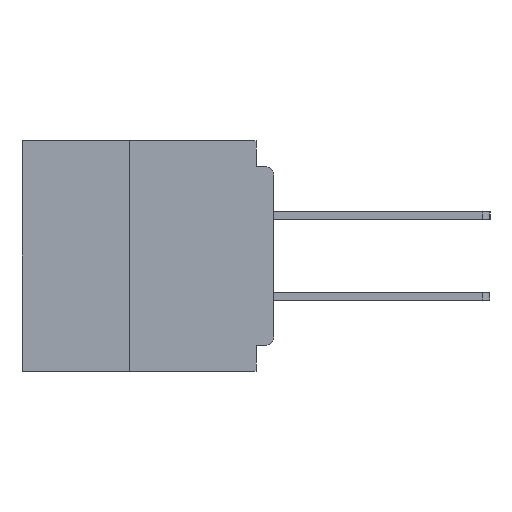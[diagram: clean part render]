
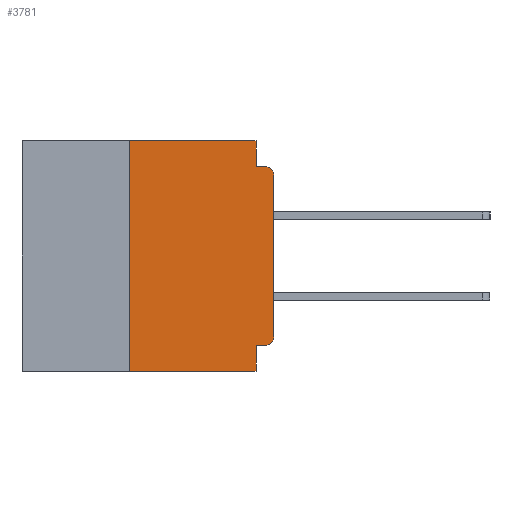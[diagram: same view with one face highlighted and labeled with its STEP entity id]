
A CAD part, left-side view. The second image highlights one B-rep face of the part: STEP entity #3781.
In plain terms, the highlighted planar face has unit normal (-1, 0, 0).
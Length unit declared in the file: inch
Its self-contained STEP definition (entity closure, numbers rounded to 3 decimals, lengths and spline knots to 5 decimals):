
#475 = LINE ( 'NONE', #21800, #40714 ) ;
#983 = DIRECTION ( 'NONE',  ( 0., -1., 0. ) ) ;
#988 = ORIENTED_EDGE ( 'NONE', *, *, #8666, .T. ) ;
#1054 = ORIENTED_EDGE ( 'NONE', *, *, #17307, .T. ) ;
#1255 = DIRECTION ( 'NONE',  ( 0., 0., -1. ) ) ;
#1446 = CARTESIAN_POINT ( 'NONE',  ( 0., 0.015, -0.34 ) ) ;
#1622 = LINE ( 'NONE', #14674, #27737 ) ;
#2168 = VERTEX_POINT ( 'NONE', #23121 ) ;
#2223 = EDGE_CURVE ( 'NONE', #4443, #34840, #23744, .T. ) ;
#2476 = ORIENTED_EDGE ( 'NONE', *, *, #20260, .F. ) ;
#3749 = CARTESIAN_POINT ( 'NONE',  ( 0., 0.031, -0.4 ) ) ;
#3781 = ADVANCED_FACE ( 'NONE', ( #30704 ), #23055, .F. ) ;
#4443 = VERTEX_POINT ( 'NONE', #14355 ) ;
#4814 = DIRECTION ( 'NONE',  ( 0., 0., -1. ) ) ;
#6836 = EDGE_CURVE ( 'NONE', #39723, #20368, #28505, .T. ) ;
#7075 = VERTEX_POINT ( 'NONE', #12648 ) ;
#7151 = AXIS2_PLACEMENT_3D ( 'NONE', #22767, #22483, #21456 ) ;
#8666 = EDGE_CURVE ( 'NONE', #13866, #19477, #31047, .T. ) ;
#10092 = VECTOR ( 'NONE', #23345, 39.37008 ) ;
#10559 = CIRCLE ( 'NONE', #15120, 0.015 ) ;
#12331 = VECTOR ( 'NONE', #38839, 39.37008 ) ;
#12599 = CARTESIAN_POINT ( 'NONE',  ( 0., 0.031, -0.045 ) ) ;
#12648 = CARTESIAN_POINT ( 'NONE',  ( 0., 0.015, -0.045 ) ) ;
#12701 = VERTEX_POINT ( 'NONE', #32894 ) ;
#13866 = VERTEX_POINT ( 'NONE', #36675 ) ;
#14355 = CARTESIAN_POINT ( 'NONE',  ( 0., 0., -0.34 ) ) ;
#14674 = CARTESIAN_POINT ( 'NONE',  ( 0., 0.25, -0.4 ) ) ;
#15120 = AXIS2_PLACEMENT_3D ( 'NONE', #1446, #24380, #4814 ) ;
#16251 = CARTESIAN_POINT ( 'NONE',  ( 0., 0.437, 0. ) ) ;
#17265 = EDGE_LOOP ( 'NONE', ( #40569, #27535, #2476, #29593, #20428, #24034, #988, #24592, #29224, #1054 ) ) ;
#17307 = EDGE_CURVE ( 'NONE', #2168, #4443, #10559, .T. ) ;
#17409 = CARTESIAN_POINT ( 'NONE',  ( 0., 0.437, -0.4 ) ) ;
#17545 = EDGE_CURVE ( 'NONE', #2168, #30224, #33842, .T. ) ;
#17609 = DIRECTION ( 'NONE',  ( 0., 0., 1. ) ) ;
#17804 = CARTESIAN_POINT ( 'NONE',  ( 0., 0., 0. ) ) ;
#18742 = LINE ( 'NONE', #3749, #10092 ) ;
#19477 = VERTEX_POINT ( 'NONE', #32264 ) ;
#20260 = EDGE_CURVE ( 'NONE', #20368, #7075, #475, .T. ) ;
#20368 = VERTEX_POINT ( 'NONE', #12599 ) ;
#20428 = ORIENTED_EDGE ( 'NONE', *, *, #30050, .F. ) ;
#20446 = CARTESIAN_POINT ( 'NONE',  ( 0., 0.031, -0.355 ) ) ;
#20901 = DIRECTION ( 'NONE',  ( -1., 0., 0. ) ) ;
#21456 = DIRECTION ( 'NONE',  ( 0., 0., -1. ) ) ;
#21800 = CARTESIAN_POINT ( 'NONE',  ( 0., 0., -0.045 ) ) ;
#21947 = LINE ( 'NONE', #16251, #12331 ) ;
#22402 = VECTOR ( 'NONE', #983, 39.37008 ) ;
#22483 = DIRECTION ( 'NONE',  ( 1., 0., 0. ) ) ;
#22767 = CARTESIAN_POINT ( 'NONE',  ( 0., 0.437, 0. ) ) ;
#23055 = PLANE ( 'NONE',  #7151 ) ;
#23121 = CARTESIAN_POINT ( 'NONE',  ( 0., 0.015, -0.355 ) ) ;
#23345 = DIRECTION ( 'NONE',  ( 0., 0., -1. ) ) ;
#23744 = LINE ( 'NONE', #17804, #33331 ) ;
#24034 = ORIENTED_EDGE ( 'NONE', *, *, #26545, .F. ) ;
#24218 = AXIS2_PLACEMENT_3D ( 'NONE', #40230, #20901, #1255 ) ;
#24380 = DIRECTION ( 'NONE',  ( -1., 0., 0. ) ) ;
#24592 = ORIENTED_EDGE ( 'NONE', *, *, #31867, .F. ) ;
#25498 = CARTESIAN_POINT ( 'NONE',  ( 0., 0., -0.355 ) ) ;
#26545 = EDGE_CURVE ( 'NONE', #13866, #12701, #1622, .T. ) ;
#27535 = ORIENTED_EDGE ( 'NONE', *, *, #40414, .T. ) ;
#27684 = CARTESIAN_POINT ( 'NONE',  ( 0., 0.031, 0. ) ) ;
#27737 = VECTOR ( 'NONE', #37281, 39.37008 ) ;
#28505 = LINE ( 'NONE', #27684, #36041 ) ;
#29224 = ORIENTED_EDGE ( 'NONE', *, *, #17545, .F. ) ;
#29593 = ORIENTED_EDGE ( 'NONE', *, *, #6836, .F. ) ;
#29956 = CARTESIAN_POINT ( 'NONE',  ( 0., 0., -0.06 ) ) ;
#30050 = EDGE_CURVE ( 'NONE', #12701, #39723, #21947, .T. ) ;
#30224 = VERTEX_POINT ( 'NONE', #20446 ) ;
#30322 = CIRCLE ( 'NONE', #24218, 0.015 ) ;
#30704 = FACE_OUTER_BOUND ( 'NONE', #17265, .T. ) ;
#31047 = LINE ( 'NONE', #17409, #22402 ) ;
#31867 = EDGE_CURVE ( 'NONE', #30224, #19477, #18742, .T. ) ;
#32004 = DIRECTION ( 'NONE',  ( 0., 1., 0. ) ) ;
#32211 = CARTESIAN_POINT ( 'NONE',  ( 0., 0.031, 0. ) ) ;
#32264 = CARTESIAN_POINT ( 'NONE',  ( 0., 0.031, -0.4 ) ) ;
#32865 = VECTOR ( 'NONE', #32004, 39.37008 ) ;
#32894 = CARTESIAN_POINT ( 'NONE',  ( 0., 0.25, 0. ) ) ;
#33331 = VECTOR ( 'NONE', #17609, 39.37008 ) ;
#33842 = LINE ( 'NONE', #25498, #32865 ) ;
#34840 = VERTEX_POINT ( 'NONE', #29956 ) ;
#36041 = VECTOR ( 'NONE', #40476, 39.37008 ) ;
#36675 = CARTESIAN_POINT ( 'NONE',  ( 0., 0.25, -0.4 ) ) ;
#37281 = DIRECTION ( 'NONE',  ( 0., 0., 1. ) ) ;
#38839 = DIRECTION ( 'NONE',  ( 0., -1., 0. ) ) ;
#39723 = VERTEX_POINT ( 'NONE', #32211 ) ;
#40230 = CARTESIAN_POINT ( 'NONE',  ( 0., 0.015, -0.06 ) ) ;
#40414 = EDGE_CURVE ( 'NONE', #34840, #7075, #30322, .T. ) ;
#40476 = DIRECTION ( 'NONE',  ( 0., 0., -1. ) ) ;
#40569 = ORIENTED_EDGE ( 'NONE', *, *, #2223, .T. ) ;
#40714 = VECTOR ( 'NONE', #41134, 39.37008 ) ;
#41134 = DIRECTION ( 'NONE',  ( 0., -1., 0. ) ) ;
